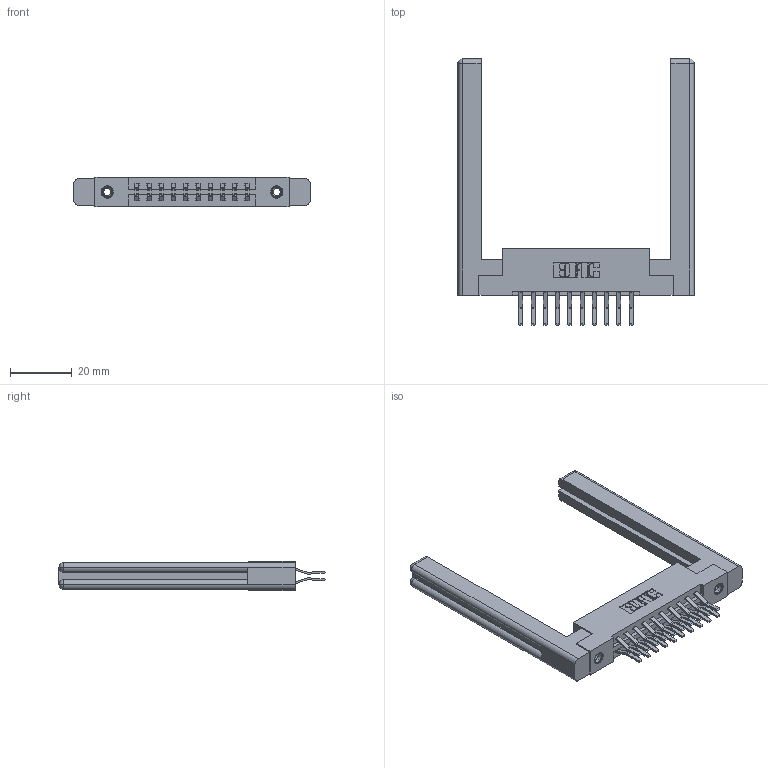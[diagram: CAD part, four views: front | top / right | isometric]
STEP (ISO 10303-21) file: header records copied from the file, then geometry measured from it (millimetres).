
FILE_DESCRIPTION (( 'STEP AP203' ), '1' );
FILE_NAME ('337-020-560-258.STEP', '2019-10-08T14:26:36', ( '' ), ( '' ), 'SwSTEP 2.0', 'SolidWorks 2016', '' );
FILE_SCHEMA (( 'CONFIG_CONTROL_DESIGN' ));
Length unit declared in the file: inch
Products named in the file (5): 307-220-058; 337 Part_Flush Mounting Lugs - 0.156 Dia-TI; 337-020-560-258; 345-250-001_345-250-001-102; 345-292-001_560 Tail
Assembly tree (25 placements, depth 2):
  337-020-560-258
    337 Part_Flush Mounting Lugs - 0.156 Dia-TI
    345-292-001_560 Tail  x20
    345-250-001_345-250-001-102  x2
    307-220-058  x2
Bounding box: 76.25 x 85.87 x 9.4 mm (x, y, z)
Volume: 14883.4 mm3; surface area: 13866.6 mm2
Topology: 25 solids, 25 shells, 1376 faces, 4005 edges, 2630 vertices
Faces by surface type: plane 914, cylinder 438, cone 12, torus 12
Entity records: 14614 total; most frequent: CARTESIAN_POINT 2497, ORIENTED_EDGE 2372, DIRECTION 2202, EDGE_CURVE 1186, LINE 1006, VECTOR 1006, VERTEX_POINT 782, AXIS2_PLACEMENT_3D 598
